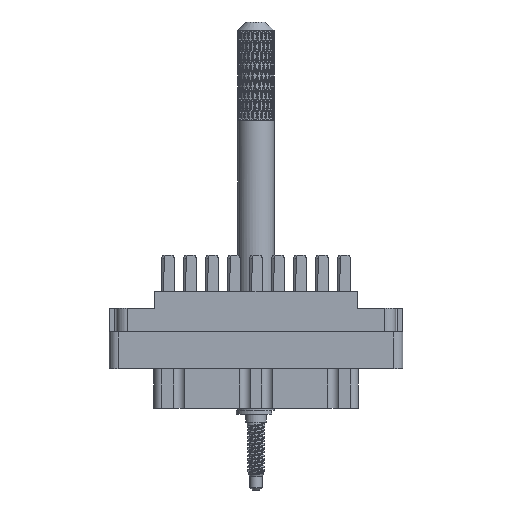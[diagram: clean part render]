
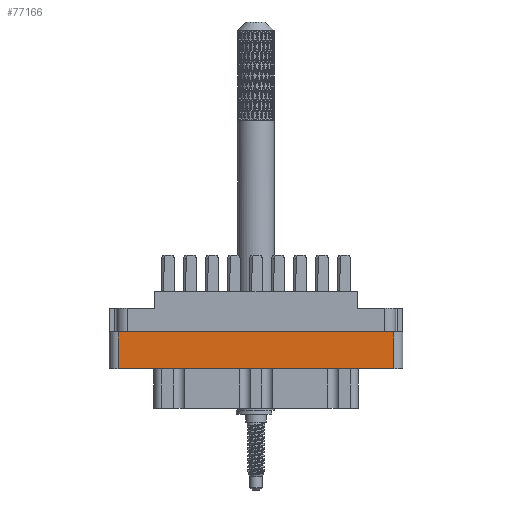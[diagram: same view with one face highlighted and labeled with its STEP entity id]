
A CAD part, front view. The second image highlights one B-rep face of the part: STEP entity #77166.
In plain terms, the highlighted planar face has unit normal (0, -1, 0).
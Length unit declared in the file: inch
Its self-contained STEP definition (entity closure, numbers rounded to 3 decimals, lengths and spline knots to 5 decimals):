
#4901 = PLANE ( 'NONE',  #29111 ) ;
#7523 = VERTEX_POINT ( 'NONE', #37113 ) ;
#15960 = ORIENTED_EDGE ( 'NONE', *, *, #94105, .F. ) ;
#16144 = LINE ( 'NONE', #78620, #46943 ) ;
#20422 = FACE_OUTER_BOUND ( 'NONE', #31592, .T. ) ;
#21419 = VERTEX_POINT ( 'NONE', #75663 ) ;
#22382 = DIRECTION ( 'NONE',  ( 0., 0., 1. ) ) ;
#24443 = DIRECTION ( 'NONE',  ( 1., 0., 0. ) ) ;
#26166 = ORIENTED_EDGE ( 'NONE', *, *, #85221, .F. ) ;
#28892 = CARTESIAN_POINT ( 'NONE',  ( 0.938, -0.438, -0.277 ) ) ;
#29111 = AXIS2_PLACEMENT_3D ( 'NONE', #74156, #82892, #66422 ) ;
#31592 = EDGE_LOOP ( 'NONE', ( #99964, #15960, #47320, #26166 ) ) ;
#31616 = VECTOR ( 'NONE', #57679, 39.37008 ) ;
#33955 = LINE ( 'NONE', #96928, #31616 ) ;
#37113 = CARTESIAN_POINT ( 'NONE',  ( 0.938, -0.438, -0.529 ) ) ;
#46943 = VECTOR ( 'NONE', #22382, 39.37008 ) ;
#47320 = ORIENTED_EDGE ( 'NONE', *, *, #99184, .T. ) ;
#54021 = CARTESIAN_POINT ( 'NONE',  ( 0.938, -0.438, -0.798 ) ) ;
#57679 = DIRECTION ( 'NONE',  ( -1., 0., 0. ) ) ;
#61271 = LINE ( 'NONE', #54021, #66502 ) ;
#65686 = VECTOR ( 'NONE', #24443, 39.37008 ) ;
#66251 = VERTEX_POINT ( 'NONE', #28892 ) ;
#66422 = DIRECTION ( 'NONE',  ( 0., 0., -1. ) ) ;
#66502 = VECTOR ( 'NONE', #77272, 39.37008 ) ;
#74156 = CARTESIAN_POINT ( 'NONE',  ( -0.938, -0.438, -0.798 ) ) ;
#75663 = CARTESIAN_POINT ( 'NONE',  ( -0.938, -0.438, -0.277 ) ) ;
#77166 = ADVANCED_FACE ( 'NONE', ( #20422 ), #4901, .T. ) ;
#77272 = DIRECTION ( 'NONE',  ( 0., 0., 1. ) ) ;
#78620 = CARTESIAN_POINT ( 'NONE',  ( -0.938, -0.438, -0.798 ) ) ;
#82307 = VERTEX_POINT ( 'NONE', #101177 ) ;
#82892 = DIRECTION ( 'NONE',  ( 0., -1., 0. ) ) ;
#85221 = EDGE_CURVE ( 'NONE', #21419, #66251, #95137, .T. ) ;
#94105 = EDGE_CURVE ( 'NONE', #7523, #82307, #33955, .T. ) ;
#95137 = LINE ( 'NONE', #95636, #65686 ) ;
#95636 = CARTESIAN_POINT ( 'NONE',  ( -1., -0.438, -0.277 ) ) ;
#96928 = CARTESIAN_POINT ( 'NONE',  ( 0.938, -0.438, -0.529 ) ) ;
#99184 = EDGE_CURVE ( 'NONE', #7523, #66251, #61271, .T. ) ;
#99964 = ORIENTED_EDGE ( 'NONE', *, *, #101816, .F. ) ;
#101177 = CARTESIAN_POINT ( 'NONE',  ( -0.938, -0.438, -0.529 ) ) ;
#101816 = EDGE_CURVE ( 'NONE', #82307, #21419, #16144, .T. ) ;
